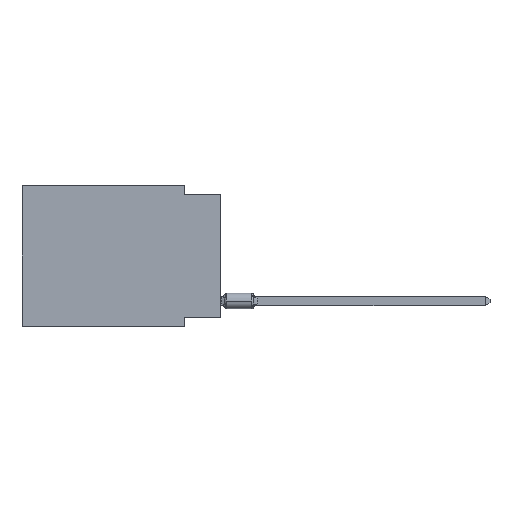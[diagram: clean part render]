
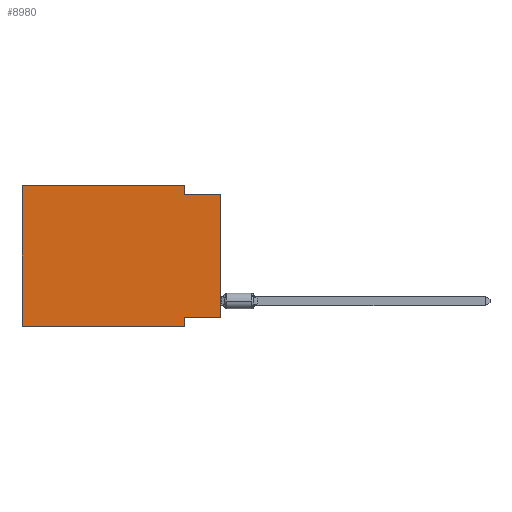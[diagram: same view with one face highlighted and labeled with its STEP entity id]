
A CAD part, left-side view. The second image highlights one B-rep face of the part: STEP entity #8980.
In plain terms, the highlighted planar face has unit normal (-1, 0, 0).
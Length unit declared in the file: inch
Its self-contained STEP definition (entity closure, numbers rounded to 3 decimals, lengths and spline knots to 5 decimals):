
#186 = ORIENTED_EDGE ( 'NONE', *, *, #12179, .F. ) ;
#258 = DIRECTION ( 'NONE',  ( 0., -1., 0. ) ) ;
#315 = LINE ( 'NONE', #10018, #10704 ) ;
#357 = EDGE_CURVE ( 'NONE', #1494, #9282, #750, .T. ) ;
#750 = LINE ( 'NONE', #12342, #3906 ) ;
#1335 = EDGE_CURVE ( 'NONE', #9282, #5468, #5656, .T. ) ;
#1356 = CARTESIAN_POINT ( 'NONE',  ( 0., 0.1, -0.025 ) ) ;
#1494 = VERTEX_POINT ( 'NONE', #11075 ) ;
#1605 = ORIENTED_EDGE ( 'NONE', *, *, #10349, .F. ) ;
#1793 = VECTOR ( 'NONE', #3139, 39.37008 ) ;
#1948 = ORIENTED_EDGE ( 'NONE', *, *, #12640, .F. ) ;
#2665 = CARTESIAN_POINT ( 'NONE',  ( 0., 0.1, -0.39 ) ) ;
#2722 = EDGE_CURVE ( 'NONE', #5650, #5468, #10928, .T. ) ;
#2847 = CARTESIAN_POINT ( 'NONE',  ( 0., 0.55, 0. ) ) ;
#2905 = VECTOR ( 'NONE', #10630, 39.37008 ) ;
#3120 = VERTEX_POINT ( 'NONE', #5796 ) ;
#3139 = DIRECTION ( 'NONE',  ( 0., 0., -1. ) ) ;
#3369 = DIRECTION ( 'NONE',  ( 1., 0., 0. ) ) ;
#3906 = VECTOR ( 'NONE', #5424, 39.37008 ) ;
#4055 = CARTESIAN_POINT ( 'NONE',  ( 0., 0., 0. ) ) ;
#4345 = PLANE ( 'NONE',  #4459 ) ;
#4459 = AXIS2_PLACEMENT_3D ( 'NONE', #12255, #3369, #7329 ) ;
#4664 = CARTESIAN_POINT ( 'NONE',  ( 0., 0., -0.025 ) ) ;
#4826 = CARTESIAN_POINT ( 'NONE',  ( 0., 0.1, -0.39 ) ) ;
#5004 = VERTEX_POINT ( 'NONE', #5771 ) ;
#5424 = DIRECTION ( 'NONE',  ( 0., 0., -1. ) ) ;
#5468 = VERTEX_POINT ( 'NONE', #8599 ) ;
#5635 = ORIENTED_EDGE ( 'NONE', *, *, #12333, .F. ) ;
#5650 = VERTEX_POINT ( 'NONE', #9040 ) ;
#5656 = LINE ( 'NONE', #4664, #2905 ) ;
#5671 = EDGE_LOOP ( 'NONE', ( #12535, #10141, #7587, #1948, #186, #10934, #1605, #5635 ) ) ;
#5771 = CARTESIAN_POINT ( 'NONE',  ( 0., 0.55, -0.39 ) ) ;
#5796 = CARTESIAN_POINT ( 'NONE',  ( 0., 0.1, -0.365 ) ) ;
#6004 = VERTEX_POINT ( 'NONE', #2665 ) ;
#6162 = CARTESIAN_POINT ( 'NONE',  ( 0., 0., -0.365 ) ) ;
#6805 = DIRECTION ( 'NONE',  ( 0., 0., 1. ) ) ;
#7142 = FACE_OUTER_BOUND ( 'NONE', #5671, .T. ) ;
#7208 = CARTESIAN_POINT ( 'NONE',  ( 0., 0.55, -0.39 ) ) ;
#7229 = VECTOR ( 'NONE', #11977, 39.37008 ) ;
#7329 = DIRECTION ( 'NONE',  ( 0., 0., -1. ) ) ;
#7587 = ORIENTED_EDGE ( 'NONE', *, *, #357, .F. ) ;
#8059 = LINE ( 'NONE', #4826, #1793 ) ;
#8599 = CARTESIAN_POINT ( 'NONE',  ( 0., 0., -0.025 ) ) ;
#8917 = EDGE_CURVE ( 'NONE', #5004, #6004, #11089, .T. ) ;
#8980 = ADVANCED_FACE ( 'NONE', ( #7142 ), #4345, .F. ) ;
#9040 = CARTESIAN_POINT ( 'NONE',  ( 0., 0., -0.365 ) ) ;
#9282 = VERTEX_POINT ( 'NONE', #1356 ) ;
#10018 = CARTESIAN_POINT ( 'NONE',  ( 0., 0.55, 0. ) ) ;
#10107 = DIRECTION ( 'NONE',  ( 0., 1., 0. ) ) ;
#10141 = ORIENTED_EDGE ( 'NONE', *, *, #1335, .F. ) ;
#10349 = EDGE_CURVE ( 'NONE', #3120, #6004, #8059, .T. ) ;
#10573 = CARTESIAN_POINT ( 'NONE',  ( 0., 0.55, 0. ) ) ;
#10630 = DIRECTION ( 'NONE',  ( 0., -1., 0. ) ) ;
#10704 = VECTOR ( 'NONE', #258, 39.37008 ) ;
#10898 = VERTEX_POINT ( 'NONE', #10573 ) ;
#10928 = LINE ( 'NONE', #4055, #7229 ) ;
#10934 = ORIENTED_EDGE ( 'NONE', *, *, #8917, .T. ) ;
#11075 = CARTESIAN_POINT ( 'NONE',  ( 0., 0.1, 0. ) ) ;
#11089 = LINE ( 'NONE', #7208, #11092 ) ;
#11092 = VECTOR ( 'NONE', #12003, 39.37008 ) ;
#11318 = VECTOR ( 'NONE', #6805, 39.37008 ) ;
#11977 = DIRECTION ( 'NONE',  ( 0., 0., 1. ) ) ;
#11993 = LINE ( 'NONE', #6162, #12352 ) ;
#12003 = DIRECTION ( 'NONE',  ( 0., -1., 0. ) ) ;
#12179 = EDGE_CURVE ( 'NONE', #5004, #10898, #12703, .T. ) ;
#12255 = CARTESIAN_POINT ( 'NONE',  ( 0., 0.55, 0. ) ) ;
#12333 = EDGE_CURVE ( 'NONE', #5650, #3120, #11993, .T. ) ;
#12342 = CARTESIAN_POINT ( 'NONE',  ( 0., 0.1, 0. ) ) ;
#12352 = VECTOR ( 'NONE', #10107, 39.37008 ) ;
#12535 = ORIENTED_EDGE ( 'NONE', *, *, #2722, .T. ) ;
#12640 = EDGE_CURVE ( 'NONE', #10898, #1494, #315, .T. ) ;
#12703 = LINE ( 'NONE', #2847, #11318 ) ;
